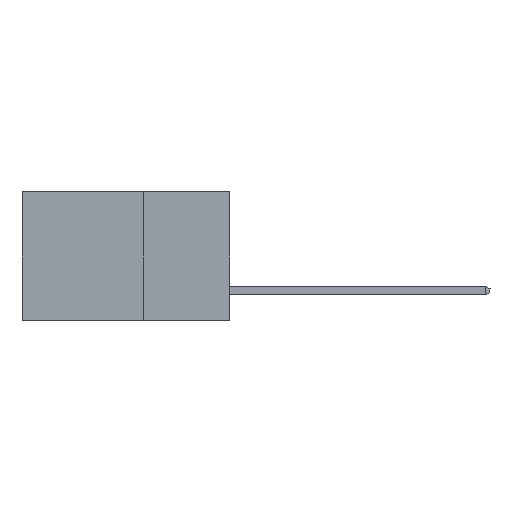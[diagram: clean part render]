
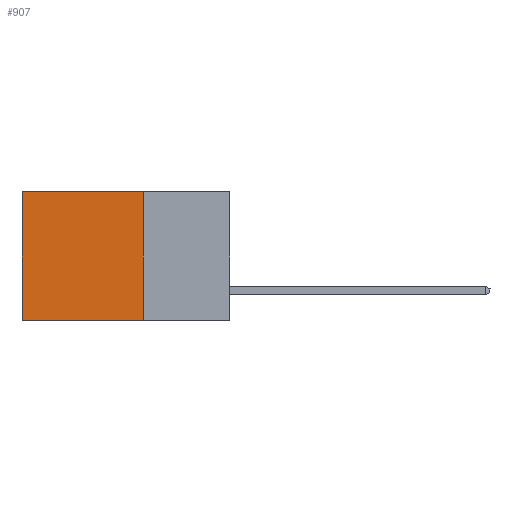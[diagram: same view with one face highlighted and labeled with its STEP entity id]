
A CAD part, left-side view. The second image highlights one B-rep face of the part: STEP entity #907.
In plain terms, the highlighted planar face has unit normal (-1, 0, 0).
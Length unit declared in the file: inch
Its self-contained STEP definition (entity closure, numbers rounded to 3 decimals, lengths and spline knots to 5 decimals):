
#581 = CARTESIAN_POINT ( 'NONE',  ( 0.2615, 0.25, 0. ) ) ;
#907 = ADVANCED_FACE ( 'NONE', ( #5604 ), #1328, .F. ) ;
#1050 = CARTESIAN_POINT ( 'NONE',  ( 0.2615, 0.25, -0.37 ) ) ;
#1097 = DIRECTION ( 'NONE',  ( 0., 0., -1. ) ) ;
#1328 = PLANE ( 'NONE',  #7271 ) ;
#1489 = ORIENTED_EDGE ( 'NONE', *, *, #3509, .F. ) ;
#1528 = CARTESIAN_POINT ( 'NONE',  ( 0.2615, 0.6, 0. ) ) ;
#1751 = CARTESIAN_POINT ( 'NONE',  ( 0.2615, 0.6, -0.37 ) ) ;
#2140 = VERTEX_POINT ( 'NONE', #1528 ) ;
#2401 = CARTESIAN_POINT ( 'NONE',  ( 0.2615, 0.25, -0.37 ) ) ;
#3081 = EDGE_LOOP ( 'NONE', ( #5647, #1489, #4846, #7954 ) ) ;
#3239 = LINE ( 'NONE', #10600, #8511 ) ;
#3509 = EDGE_CURVE ( 'NONE', #10062, #10154, #7439, .T. ) ;
#3715 = VECTOR ( 'NONE', #9184, 39.37008 ) ;
#4693 = VERTEX_POINT ( 'NONE', #581 ) ;
#4846 = ORIENTED_EDGE ( 'NONE', *, *, #10110, .F. ) ;
#5037 = LINE ( 'NONE', #8523, #3715 ) ;
#5368 = EDGE_CURVE ( 'NONE', #4693, #2140, #3239, .T. ) ;
#5407 = VECTOR ( 'NONE', #6392, 39.37008 ) ;
#5604 = FACE_OUTER_BOUND ( 'NONE', #3081, .T. ) ;
#5647 = ORIENTED_EDGE ( 'NONE', *, *, #7178, .T. ) ;
#6392 = DIRECTION ( 'NONE',  ( 0., 1., 0. ) ) ;
#6597 = DIRECTION ( 'NONE',  ( 1., 0., 0. ) ) ;
#7178 = EDGE_CURVE ( 'NONE', #2140, #10154, #5037, .T. ) ;
#7271 = AXIS2_PLACEMENT_3D ( 'NONE', #10673, #6597, #9044 ) ;
#7439 = LINE ( 'NONE', #2401, #5407 ) ;
#7656 = CARTESIAN_POINT ( 'NONE',  ( 0.2615, 0.25, -0.37 ) ) ;
#7954 = ORIENTED_EDGE ( 'NONE', *, *, #5368, .T. ) ;
#8511 = VECTOR ( 'NONE', #9901, 39.37008 ) ;
#8523 = CARTESIAN_POINT ( 'NONE',  ( 0.2615, 0.6, -0.37 ) ) ;
#9044 = DIRECTION ( 'NONE',  ( 0., 0., -1. ) ) ;
#9184 = DIRECTION ( 'NONE',  ( 0., 0., -1. ) ) ;
#9658 = VECTOR ( 'NONE', #1097, 39.37008 ) ;
#9901 = DIRECTION ( 'NONE',  ( 0., 1., 0. ) ) ;
#10062 = VERTEX_POINT ( 'NONE', #1050 ) ;
#10089 = LINE ( 'NONE', #7656, #9658 ) ;
#10110 = EDGE_CURVE ( 'NONE', #4693, #10062, #10089, .T. ) ;
#10154 = VERTEX_POINT ( 'NONE', #1751 ) ;
#10600 = CARTESIAN_POINT ( 'NONE',  ( 0.2615, 0.25, 0. ) ) ;
#10673 = CARTESIAN_POINT ( 'NONE',  ( 0.2615, 0.25, -0.37 ) ) ;
